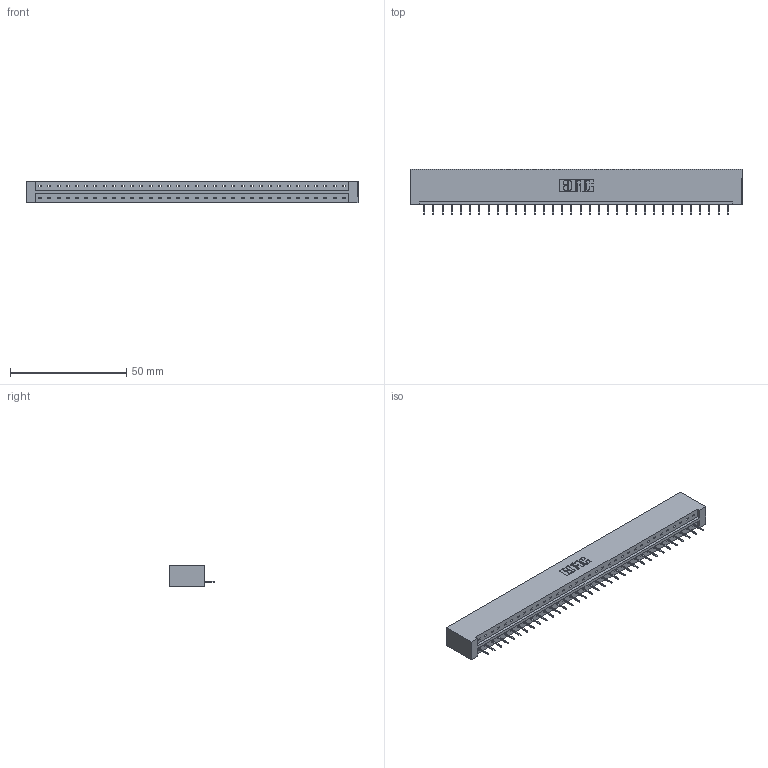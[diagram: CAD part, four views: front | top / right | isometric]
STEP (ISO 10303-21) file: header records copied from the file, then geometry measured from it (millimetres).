
FILE_DESCRIPTION (( 'STEP AP203' ), '1' );
FILE_NAME ('333-034-524-101.STEP', '2018-08-02T22:05:15', ( '' ), ( '' ), 'SwSTEP 2.0', 'SolidWorks 2016', '' );
FILE_SCHEMA (( 'CONFIG_CONTROL_DESIGN' ));
Length unit declared in the file: inch
Products named in the file (3): 333 Part_Lugless; 345-292-001_345-293-124; 333-034-524-101
Assembly tree (35 placements, depth 2):
  333-034-524-101
    333 Part_Lugless
    345-292-001_345-293-124  x34
Bounding box: 142.98 x 19.69 x 9.4 mm (x, y, z)
Volume: 14797.1 mm3; surface area: 15452.8 mm2
Topology: 35 solids, 35 shells, 2214 faces, 6407 edges, 4134 vertices
Faces by surface type: plane 1698, cylinder 516
Entity records: 21617 total; most frequent: CARTESIAN_POINT 3736, ORIENTED_EDGE 3706, DIRECTION 3161, EDGE_CURVE 1853, VECTOR 1737, LINE 1737, VERTEX_POINT 1230, AXIS2_PLACEMENT_3D 712
